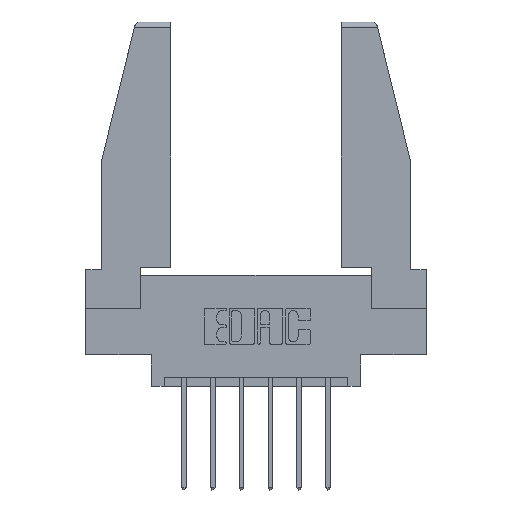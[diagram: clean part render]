
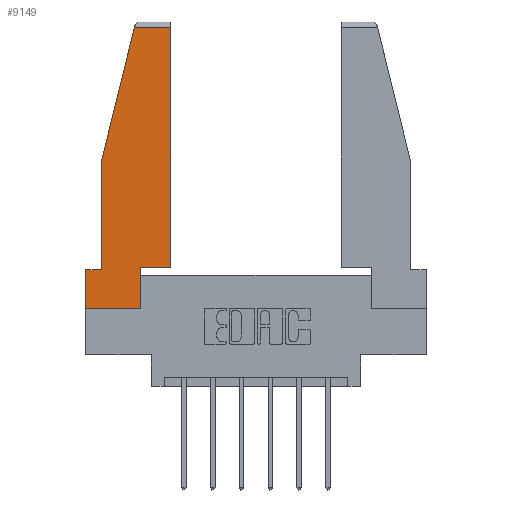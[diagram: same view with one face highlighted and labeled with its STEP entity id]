
A CAD part, top view. The second image highlights one B-rep face of the part: STEP entity #9149.
In plain terms, the highlighted planar face has unit normal (0, 0, 1).
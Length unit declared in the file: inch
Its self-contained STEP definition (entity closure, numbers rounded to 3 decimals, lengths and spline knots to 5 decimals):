
#276 = VECTOR ( 'NONE', #870, 39.37008 ) ;
#435 = DIRECTION ( 'NONE',  ( 1., 0., 0. ) ) ;
#631 = DIRECTION ( 'NONE',  ( 0., 1., 0. ) ) ;
#697 = CARTESIAN_POINT ( 'NONE',  ( 0.461, 1.52, 0. ) ) ;
#804 = LINE ( 'NONE', #1317, #11193 ) ;
#870 = DIRECTION ( 'NONE',  ( -1., 0., 0. ) ) ;
#1317 = CARTESIAN_POINT ( 'NONE',  ( 0.086, 0.8, 0. ) ) ;
#1516 = VECTOR ( 'NONE', #631, 39.37008 ) ;
#1785 = EDGE_CURVE ( 'NONE', #3021, #1902, #804, .T. ) ;
#1800 = EDGE_CURVE ( 'NONE', #3158, #4065, #5723, .T. ) ;
#1864 = CARTESIAN_POINT ( 'NONE',  ( 0., 0., 0. ) ) ;
#1902 = VERTEX_POINT ( 'NONE', #9440 ) ;
#2035 = EDGE_CURVE ( 'NONE', #4065, #3992, #3566, .T. ) ;
#2204 = CARTESIAN_POINT ( 'NONE',  ( 0.297, 0.223, 0. ) ) ;
#2219 = LINE ( 'NONE', #2262, #6861 ) ;
#2262 = CARTESIAN_POINT ( 'NONE',  ( 0.271, 1.55, 0. ) ) ;
#2609 = CARTESIAN_POINT ( 'NONE',  ( 0., 0., 0. ) ) ;
#2744 = EDGE_CURVE ( 'NONE', #3992, #7800, #11304, .T. ) ;
#2849 = ORIENTED_EDGE ( 'NONE', *, *, #7515, .T. ) ;
#3021 = VERTEX_POINT ( 'NONE', #3749 ) ;
#3158 = VERTEX_POINT ( 'NONE', #2204 ) ;
#3325 = ORIENTED_EDGE ( 'NONE', *, *, #2035, .T. ) ;
#3396 = CARTESIAN_POINT ( 'NONE',  ( 0.461, 0.223, 0. ) ) ;
#3566 = LINE ( 'NONE', #3396, #1516 ) ;
#3749 = CARTESIAN_POINT ( 'NONE',  ( 0.086, 0.8, 0. ) ) ;
#3992 = VERTEX_POINT ( 'NONE', #697 ) ;
#4065 = VERTEX_POINT ( 'NONE', #9150 ) ;
#4124 = DIRECTION ( 'NONE',  ( 0., 1., 0. ) ) ;
#4207 = LINE ( 'NONE', #5148, #10846 ) ;
#4212 = CARTESIAN_POINT ( 'NONE',  ( 0.297, 0., 0. ) ) ;
#4907 = ORIENTED_EDGE ( 'NONE', *, *, #2744, .T. ) ;
#4924 = EDGE_CURVE ( 'NONE', #7800, #3021, #2219, .T. ) ;
#5148 = CARTESIAN_POINT ( 'NONE',  ( 0., 0.21, 0. ) ) ;
#5282 = VECTOR ( 'NONE', #10629, 39.37008 ) ;
#5492 = PLANE ( 'NONE',  #11420 ) ;
#5563 = CARTESIAN_POINT ( 'NONE',  ( 0., 0., 0. ) ) ;
#5723 = LINE ( 'NONE', #6940, #8737 ) ;
#5743 = LINE ( 'NONE', #4212, #6757 ) ;
#6266 = DIRECTION ( 'NONE',  ( 0., -1., 0. ) ) ;
#6642 = ORIENTED_EDGE ( 'NONE', *, *, #4924, .T. ) ;
#6757 = VECTOR ( 'NONE', #4124, 39.37008 ) ;
#6861 = VECTOR ( 'NONE', #7006, 39.37008 ) ;
#6940 = CARTESIAN_POINT ( 'NONE',  ( 0.297, 0.223, 0. ) ) ;
#7006 = DIRECTION ( 'NONE',  ( -0.239, -0.971, 0. ) ) ;
#7465 = DIRECTION ( 'NONE',  ( 1., 0., 0. ) ) ;
#7515 = EDGE_CURVE ( 'NONE', #7839, #9183, #4207, .T. ) ;
#7722 = CARTESIAN_POINT ( 'NONE',  ( 0., 0.21, 0. ) ) ;
#7800 = VERTEX_POINT ( 'NONE', #11525 ) ;
#7839 = VERTEX_POINT ( 'NONE', #7722 ) ;
#8091 = EDGE_CURVE ( 'NONE', #1902, #7839, #9807, .T. ) ;
#8200 = FACE_OUTER_BOUND ( 'NONE', #11882, .T. ) ;
#8640 = VERTEX_POINT ( 'NONE', #11177 ) ;
#8737 = VECTOR ( 'NONE', #435, 39.37008 ) ;
#8829 = LINE ( 'NONE', #1864, #10553 ) ;
#8867 = ORIENTED_EDGE ( 'NONE', *, *, #11040, .T. ) ;
#8976 = EDGE_CURVE ( 'NONE', #8640, #3158, #5743, .T. ) ;
#9149 = ADVANCED_FACE ( 'NONE', ( #8200 ), #5492, .T. ) ;
#9150 = CARTESIAN_POINT ( 'NONE',  ( 0.461, 0.223, 0. ) ) ;
#9183 = VERTEX_POINT ( 'NONE', #5563 ) ;
#9185 = ORIENTED_EDGE ( 'NONE', *, *, #1785, .T. ) ;
#9440 = CARTESIAN_POINT ( 'NONE',  ( 0.086, 0.21, 0. ) ) ;
#9589 = CARTESIAN_POINT ( 'NONE',  ( 0., 1.52, 0. ) ) ;
#9707 = ORIENTED_EDGE ( 'NONE', *, *, #8976, .T. ) ;
#9807 = LINE ( 'NONE', #11750, #276 ) ;
#9960 = ORIENTED_EDGE ( 'NONE', *, *, #1800, .T. ) ;
#10473 = ORIENTED_EDGE ( 'NONE', *, *, #8091, .T. ) ;
#10553 = VECTOR ( 'NONE', #7465, 39.37008 ) ;
#10629 = DIRECTION ( 'NONE',  ( -1., 0., 0. ) ) ;
#10846 = VECTOR ( 'NONE', #11617, 39.37008 ) ;
#11040 = EDGE_CURVE ( 'NONE', #9183, #8640, #8829, .T. ) ;
#11177 = CARTESIAN_POINT ( 'NONE',  ( 0.297, 0., 0. ) ) ;
#11193 = VECTOR ( 'NONE', #6266, 39.37008 ) ;
#11304 = LINE ( 'NONE', #9589, #5282 ) ;
#11420 = AXIS2_PLACEMENT_3D ( 'NONE', #2609, #11830, #11897 ) ;
#11525 = CARTESIAN_POINT ( 'NONE',  ( 0.2636, 1.52, 0. ) ) ;
#11617 = DIRECTION ( 'NONE',  ( 0., -1., 0. ) ) ;
#11750 = CARTESIAN_POINT ( 'NONE',  ( 0., 0.21, 0. ) ) ;
#11830 = DIRECTION ( 'NONE',  ( 0., 0., 1. ) ) ;
#11882 = EDGE_LOOP ( 'NONE', ( #3325, #4907, #6642, #9185, #10473, #2849, #8867, #9707, #9960 ) ) ;
#11897 = DIRECTION ( 'NONE',  ( 1., 0., 0. ) ) ;
